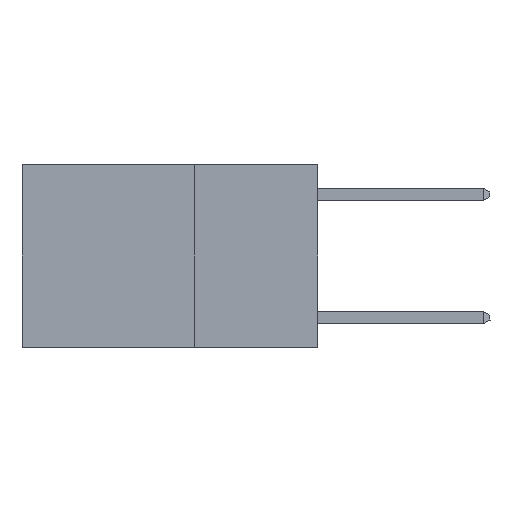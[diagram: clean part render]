
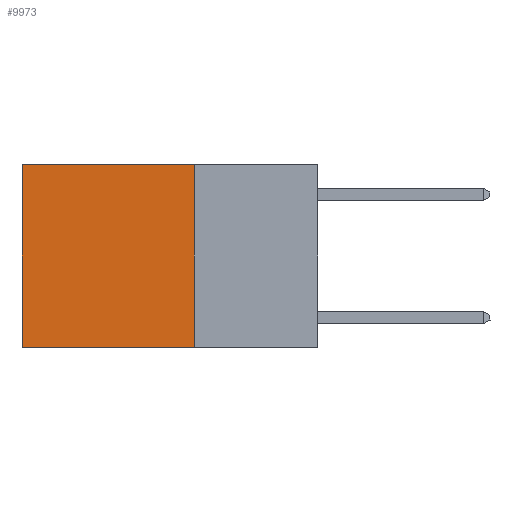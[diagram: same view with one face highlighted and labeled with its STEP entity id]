
A CAD part, left-side view. The second image highlights one B-rep face of the part: STEP entity #9973.
In plain terms, the highlighted planar face has unit normal (-1, 0, 0).
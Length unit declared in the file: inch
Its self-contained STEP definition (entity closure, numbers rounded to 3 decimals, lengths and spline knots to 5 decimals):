
#1061 = PLANE ( 'NONE',  #6805 ) ;
#1143 = DIRECTION ( 'NONE',  ( 1., 0., 0. ) ) ;
#2924 = DIRECTION ( 'NONE',  ( 0., 1., 0. ) ) ;
#3333 = DIRECTION ( 'NONE',  ( 0., 0., -1. ) ) ;
#3603 = EDGE_LOOP ( 'NONE', ( #14465, #21319, #13477, #4731 ) ) ;
#4215 = LINE ( 'NONE', #10388, #22313 ) ;
#4219 = LINE ( 'NONE', #11680, #17782 ) ;
#4731 = ORIENTED_EDGE ( 'NONE', *, *, #5066, .T. ) ;
#4874 = CARTESIAN_POINT ( 'NONE',  ( 0.2625, 0.6, 0. ) ) ;
#5066 = EDGE_CURVE ( 'NONE', #14860, #16029, #22625, .T. ) ;
#6805 = AXIS2_PLACEMENT_3D ( 'NONE', #11776, #1143, #13573 ) ;
#7404 = LINE ( 'NONE', #4874, #20787 ) ;
#8724 = VECTOR ( 'NONE', #10810, 39.37008 ) ;
#9843 = CARTESIAN_POINT ( 'NONE',  ( 0.2625, 0.25, -0.37 ) ) ;
#9973 = ADVANCED_FACE ( 'NONE', ( #21063 ), #1061, .F. ) ;
#10388 = CARTESIAN_POINT ( 'NONE',  ( 0.2625, 0.25, 0. ) ) ;
#10639 = VERTEX_POINT ( 'NONE', #9843 ) ;
#10810 = DIRECTION ( 'NONE',  ( 0., 1., 0. ) ) ;
#11680 = CARTESIAN_POINT ( 'NONE',  ( 0.2625, 0.25, -0.37 ) ) ;
#11776 = CARTESIAN_POINT ( 'NONE',  ( 0.2625, 0.25, 0. ) ) ;
#12241 = EDGE_CURVE ( 'NONE', #14860, #10639, #4215, .T. ) ;
#13477 = ORIENTED_EDGE ( 'NONE', *, *, #12241, .F. ) ;
#13573 = DIRECTION ( 'NONE',  ( 0., 0., -1. ) ) ;
#14032 = EDGE_CURVE ( 'NONE', #10639, #14248, #4219, .T. ) ;
#14248 = VERTEX_POINT ( 'NONE', #21502 ) ;
#14465 = ORIENTED_EDGE ( 'NONE', *, *, #20678, .T. ) ;
#14860 = VERTEX_POINT ( 'NONE', #19574 ) ;
#15664 = CARTESIAN_POINT ( 'NONE',  ( 0.2625, 0.6, 0. ) ) ;
#16029 = VERTEX_POINT ( 'NONE', #15664 ) ;
#16130 = CARTESIAN_POINT ( 'NONE',  ( 0.2625, 0.25, 0. ) ) ;
#17259 = DIRECTION ( 'NONE',  ( 0., 0., -1. ) ) ;
#17782 = VECTOR ( 'NONE', #2924, 39.37008 ) ;
#19574 = CARTESIAN_POINT ( 'NONE',  ( 0.2625, 0.25, 0. ) ) ;
#20678 = EDGE_CURVE ( 'NONE', #16029, #14248, #7404, .T. ) ;
#20787 = VECTOR ( 'NONE', #17259, 39.37008 ) ;
#21063 = FACE_OUTER_BOUND ( 'NONE', #3603, .T. ) ;
#21319 = ORIENTED_EDGE ( 'NONE', *, *, #14032, .F. ) ;
#21502 = CARTESIAN_POINT ( 'NONE',  ( 0.2625, 0.6, -0.37 ) ) ;
#22313 = VECTOR ( 'NONE', #3333, 39.37008 ) ;
#22625 = LINE ( 'NONE', #16130, #8724 ) ;
